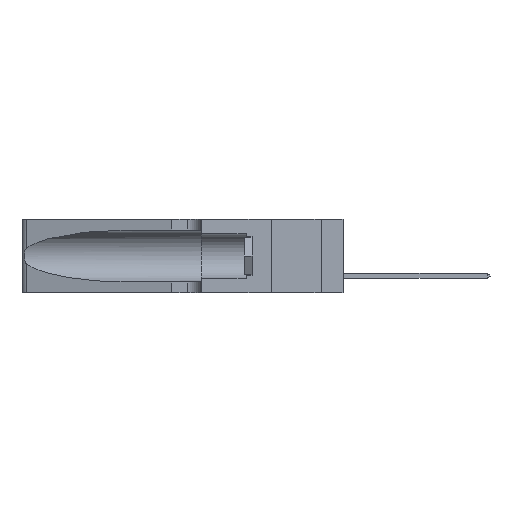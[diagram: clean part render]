
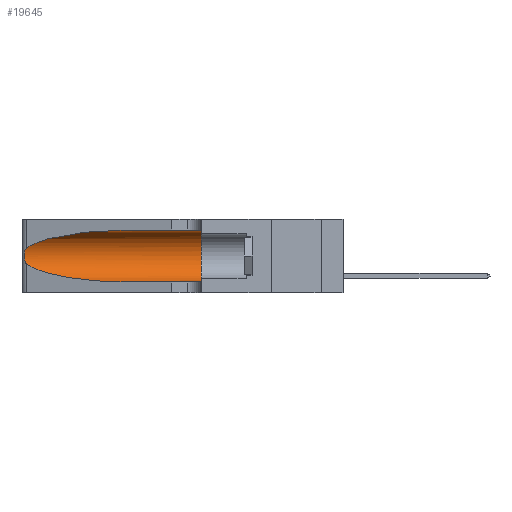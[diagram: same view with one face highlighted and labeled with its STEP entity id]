
A CAD part, left-side view. The second image highlights one B-rep face of the part: STEP entity #19645.
In plain terms, the highlighted cylindrical face has radius 3.308 mm (diameter 6.617 mm), a partial arc.
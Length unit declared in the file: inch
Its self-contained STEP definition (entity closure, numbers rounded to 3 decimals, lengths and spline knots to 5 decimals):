
#165 = CARTESIAN_POINT ( 'NONE',  ( 0.25487, 1.22718, 0.22369 ) ) ;
#488 = ORIENTED_EDGE ( 'NONE', *, *, #11616, .F. ) ;
#587 = CARTESIAN_POINT ( 'NONE',  ( 0.25856, 1.23593, 0.16098 ) ) ;
#805 = CARTESIAN_POINT ( 'NONE',  ( 0.18966, 0.96281, 0.05475 ) ) ;
#1095 = ORIENTED_EDGE ( 'NONE', *, *, #9075, .T. ) ;
#1158 = VERTEX_POINT ( 'NONE', #21124 ) ;
#1738 = CARTESIAN_POINT ( 'NONE',  ( 0.1305, 0.72297, 0.05475 ) ) ;
#2210 =( BOUNDED_CURVE ( )  B_SPLINE_CURVE ( 3, ( #6989, #15794, #7060, #19335 ),
 .UNSPECIFIED., .F., .T. ) 
 B_SPLINE_CURVE_WITH_KNOTS ( ( 4, 4 ),
 ( 1.5708, 2.84003 ),
 .UNSPECIFIED. ) 
 CURVE ( )  GEOMETRIC_REPRESENTATION_ITEM ( )  RATIONAL_B_SPLINE_CURVE ( ( 1., 0.87, 0.87, 1. ) ) 
 REPRESENTATION_ITEM ( '' )  );
#2441 = CARTESIAN_POINT ( 'NONE',  ( 0.25639, 1.23184, 0.21858 ) ) ;
#2526 = CARTESIAN_POINT ( 'NONE',  ( 0.25487, 1.22718, 0.14631 ) ) ;
#3513 = EDGE_CURVE ( 'NONE', #15047, #14558, #2210, .T. ) ;
#3547 = CARTESIAN_POINT ( 'NONE',  ( 0.25487, 1.22718, 0.22369 ) ) ;
#4114 = ORIENTED_EDGE ( 'NONE', *, *, #18386, .T. ) ;
#4625 = CARTESIAN_POINT ( 'NONE',  ( 0.1305, 1.61858, 0.05475 ) ) ;
#5045 = VERTEX_POINT ( 'NONE', #19916 ) ;
#5237 = EDGE_CURVE ( 'NONE', #9265, #1158, #9002, .T. ) ;
#5308 = AXIS2_PLACEMENT_3D ( 'NONE', #11777, #6181, #9796 ) ;
#5315 = B_SPLINE_CURVE_WITH_KNOTS ( 'NONE', 3,
 ( #165, #9129, #2441, #5843, #16485, #21641, #14884, #5988, #7746, #587, #13037, #7671, #18411, #2526 ),
 .UNSPECIFIED., .F., .F.,
 ( 4, 2, 2, 2, 2, 2, 4 ),
 ( 0., 0.00027, 0.00053, 0.00107, 0.0016, 0.00187, 0.00214 ),
 .UNSPECIFIED. ) ;
#5843 = CARTESIAN_POINT ( 'NONE',  ( 0.25787, 1.23484, 0.2124 ) ) ;
#5988 = CARTESIAN_POINT ( 'NONE',  ( 0.26075, 1.23896, 0.178 ) ) ;
#6181 = DIRECTION ( 'NONE',  ( 0., -1., 0. ) ) ;
#6429 = CARTESIAN_POINT ( 'NONE',  ( 0.1305, 1.61858, 0.31525 ) ) ;
#6989 = CARTESIAN_POINT ( 'NONE',  ( 0.1305, 0.72297, 0.31525 ) ) ;
#7060 = CARTESIAN_POINT ( 'NONE',  ( 0.2373, 1.15595, 0.28018 ) ) ;
#7671 = CARTESIAN_POINT ( 'NONE',  ( 0.25639, 1.23186, 0.15144 ) ) ;
#7746 = CARTESIAN_POINT ( 'NONE',  ( 0.26017, 1.23833, 0.17102 ) ) ;
#7889 = CARTESIAN_POINT ( 'NONE',  ( 0.1305, 0.72297, 0.05475 ) ) ;
#7925 = ORIENTED_EDGE ( 'NONE', *, *, #3513, .T. ) ;
#8012 = ORIENTED_EDGE ( 'NONE', *, *, #20444, .T. ) ;
#8597 = DIRECTION ( 'NONE',  ( 0., 0., 1. ) ) ;
#9002 = CIRCLE ( 'NONE', #12043, 0.13025 ) ;
#9075 = EDGE_CURVE ( 'NONE', #14558, #5045, #5315, .T. ) ;
#9105 = CARTESIAN_POINT ( 'NONE',  ( 0.1305, 0.72297, 0.31525 ) ) ;
#9129 = CARTESIAN_POINT ( 'NONE',  ( 0.25555, 1.22994, 0.2215 ) ) ;
#9265 = VERTEX_POINT ( 'NONE', #9653 ) ;
#9631 = VERTEX_POINT ( 'NONE', #1738 ) ;
#9653 = CARTESIAN_POINT ( 'NONE',  ( 0.1305, 0.35, 0.31525 ) ) ;
#9796 = DIRECTION ( 'NONE',  ( 0., 0., -1. ) ) ;
#11375 = VECTOR ( 'NONE', #16343, 39.37008 ) ;
#11513 = DIRECTION ( 'NONE',  ( 0., -1., 0. ) ) ;
#11616 = EDGE_CURVE ( 'NONE', #15047, #9265, #17416, .T. ) ;
#11777 = CARTESIAN_POINT ( 'NONE',  ( 0.1305, 1.61858, 0.185 ) ) ;
#12043 = AXIS2_PLACEMENT_3D ( 'NONE', #20865, #17269, #8597 ) ;
#13037 = CARTESIAN_POINT ( 'NONE',  ( 0.25789, 1.23486, 0.15765 ) ) ;
#13258 = LINE ( 'NONE', #4625, #11375 ) ;
#14107 = FACE_OUTER_BOUND ( 'NONE', #18336, .T. ) ;
#14380 = CARTESIAN_POINT ( 'NONE',  ( 0.25487, 1.22718, 0.14631 ) ) ;
#14558 = VERTEX_POINT ( 'NONE', #3547 ) ;
#14884 = CARTESIAN_POINT ( 'NONE',  ( 0.26075, 1.23896, 0.19203 ) ) ;
#15047 = VERTEX_POINT ( 'NONE', #9105 ) ;
#15794 = CARTESIAN_POINT ( 'NONE',  ( 0.18966, 0.96281, 0.31525 ) ) ;
#16155 = CARTESIAN_POINT ( 'NONE',  ( 0.2373, 1.15595, 0.08982 ) ) ;
#16343 = DIRECTION ( 'NONE',  ( 0., -1., 0. ) ) ;
#16485 = CARTESIAN_POINT ( 'NONE',  ( 0.25854, 1.2359, 0.20912 ) ) ;
#16941 = ORIENTED_EDGE ( 'NONE', *, *, #5237, .F. ) ;
#17269 = DIRECTION ( 'NONE',  ( 0., 1., 0. ) ) ;
#17416 = LINE ( 'NONE', #6429, #22390 ) ;
#18336 = EDGE_LOOP ( 'NONE', ( #7925, #1095, #4114, #8012, #16941, #488 ) ) ;
#18386 = EDGE_CURVE ( 'NONE', #5045, #9631, #18954, .T. ) ;
#18411 = CARTESIAN_POINT ( 'NONE',  ( 0.25555, 1.22993, 0.14849 ) ) ;
#18799 = CYLINDRICAL_SURFACE ( 'NONE', #5308, 0.13025 ) ;
#18954 =( BOUNDED_CURVE ( )  B_SPLINE_CURVE ( 3, ( #14380, #16155, #805, #7889 ),
 .UNSPECIFIED., .F., .F. ) 
 B_SPLINE_CURVE_WITH_KNOTS ( ( 4, 4 ),
 ( 3.44316, 4.71239 ),
 .UNSPECIFIED. ) 
 CURVE ( )  GEOMETRIC_REPRESENTATION_ITEM ( )  RATIONAL_B_SPLINE_CURVE ( ( 1., 0.87, 0.87, 1. ) ) 
 REPRESENTATION_ITEM ( '' )  );
#19335 = CARTESIAN_POINT ( 'NONE',  ( 0.25487, 1.22718, 0.22369 ) ) ;
#19645 = ADVANCED_FACE ( 'NONE', ( #14107 ), #18799, .F. ) ;
#19916 = CARTESIAN_POINT ( 'NONE',  ( 0.25487, 1.22718, 0.14631 ) ) ;
#20444 = EDGE_CURVE ( 'NONE', #9631, #1158, #13258, .T. ) ;
#20865 = CARTESIAN_POINT ( 'NONE',  ( 0.1305, 0.35, 0.185 ) ) ;
#21124 = CARTESIAN_POINT ( 'NONE',  ( 0.1305, 0.35, 0.05475 ) ) ;
#21641 = CARTESIAN_POINT ( 'NONE',  ( 0.26018, 1.23835, 0.19895 ) ) ;
#22390 = VECTOR ( 'NONE', #11513, 39.37008 ) ;
